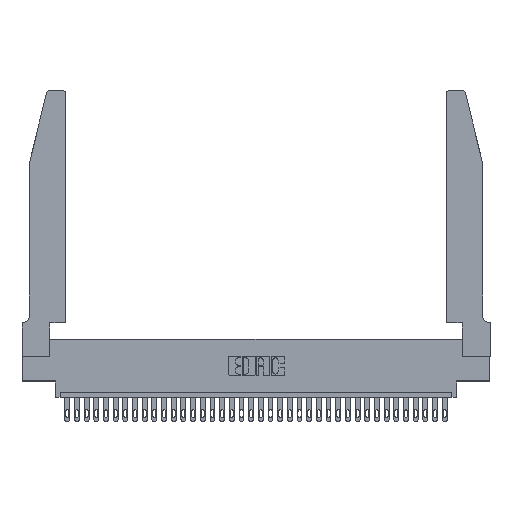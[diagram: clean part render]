
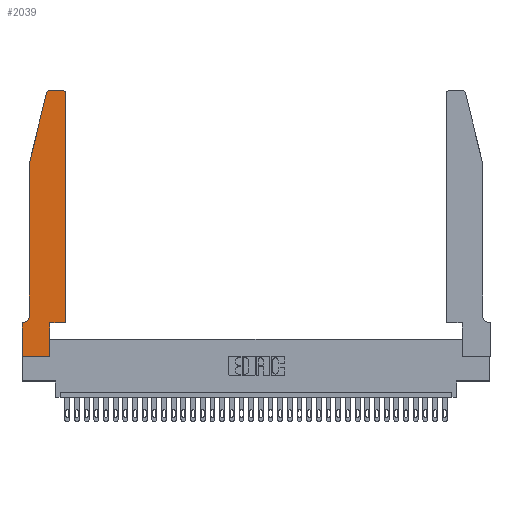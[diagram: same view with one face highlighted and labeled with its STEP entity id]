
A CAD part, top view. The second image highlights one B-rep face of the part: STEP entity #2039.
In plain terms, the highlighted planar face has unit normal (0, 0, 1).
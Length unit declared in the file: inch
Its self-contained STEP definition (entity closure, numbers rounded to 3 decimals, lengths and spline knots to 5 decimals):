
#316 = LINE ( 'NONE', #12608, #26668 ) ;
#741 = DIRECTION ( 'NONE',  ( 1., 0., 0. ) ) ;
#798 = DIRECTION ( 'NONE',  ( 0., 0., 1. ) ) ;
#1268 = VERTEX_POINT ( 'NONE', #8840 ) ;
#2039 = ADVANCED_FACE ( 'NONE', ( #13222 ), #33910, .T. ) ;
#2262 = EDGE_CURVE ( 'NONE', #23707, #23118, #3059, .T. ) ;
#2344 = CARTESIAN_POINT ( 'NONE',  ( 0.4505, 2.72, 0.37 ) ) ;
#2407 = CIRCLE ( 'NONE', #11731, 0.03 ) ;
#2516 = LINE ( 'NONE', #16921, #28808 ) ;
#2754 = EDGE_CURVE ( 'NONE', #29681, #28949, #15750, .T. ) ;
#2791 = ORIENTED_EDGE ( 'NONE', *, *, #12089, .T. ) ;
#2829 = CARTESIAN_POINT ( 'NONE',  ( 0., 0., 0.37 ) ) ;
#3059 = LINE ( 'NONE', #30527, #8102 ) ;
#4511 = LINE ( 'NONE', #7161, #32981 ) ;
#4590 = DIRECTION ( 'NONE',  ( 0., 0., 1. ) ) ;
#4841 = EDGE_CURVE ( 'NONE', #22587, #20092, #33483, .T. ) ;
#7075 = DIRECTION ( 'NONE',  ( 1., 0., 0. ) ) ;
#7161 = CARTESIAN_POINT ( 'NONE',  ( 0., 0., 0.37 ) ) ;
#8011 = DIRECTION ( 'NONE',  ( -1., 0., 0. ) ) ;
#8050 = VERTEX_POINT ( 'NONE', #22201 ) ;
#8102 = VECTOR ( 'NONE', #741, 39.37008 ) ;
#8840 = CARTESIAN_POINT ( 'NONE',  ( 0.0055, 0.35, 0.37 ) ) ;
#9217 = DIRECTION ( 'NONE',  ( 1., 0., 0. ) ) ;
#10300 = VERTEX_POINT ( 'NONE', #2829 ) ;
#10468 = ORIENTED_EDGE ( 'NONE', *, *, #2262, .T. ) ;
#10842 = EDGE_CURVE ( 'NONE', #23118, #29681, #2516, .T. ) ;
#10985 = ORIENTED_EDGE ( 'NONE', *, *, #14538, .T. ) ;
#11731 = AXIS2_PLACEMENT_3D ( 'NONE', #12635, #4590, #7075 ) ;
#12049 = CARTESIAN_POINT ( 'NONE',  ( 0., 0.35, 0.37 ) ) ;
#12089 = EDGE_CURVE ( 'NONE', #10300, #8050, #4511, .T. ) ;
#12608 = CARTESIAN_POINT ( 'NONE',  ( 0.2865, 0.35, 0.37 ) ) ;
#12635 = CARTESIAN_POINT ( 'NONE',  ( 0.284, 2.72, 0.37 ) ) ;
#12711 = VECTOR ( 'NONE', #31027, 39.37008 ) ;
#12812 = VERTEX_POINT ( 'NONE', #15108 ) ;
#13222 = FACE_OUTER_BOUND ( 'NONE', #23418, .T. ) ;
#14308 = CARTESIAN_POINT ( 'NONE',  ( 0.0755, 2., 0.37 ) ) ;
#14431 = LINE ( 'NONE', #31147, #12711 ) ;
#14538 = EDGE_CURVE ( 'NONE', #28949, #34272, #14431, .T. ) ;
#14582 = CARTESIAN_POINT ( 'NONE',  ( 0.4505, 0.35, 0.37 ) ) ;
#15108 = CARTESIAN_POINT ( 'NONE',  ( 0.25487, 2.72718, 0.37 ) ) ;
#15146 = DIRECTION ( 'NONE',  ( 1., 0., 0. ) ) ;
#15150 = ORIENTED_EDGE ( 'NONE', *, *, #21314, .T. ) ;
#15430 = ORIENTED_EDGE ( 'NONE', *, *, #10842, .T. ) ;
#15750 = CIRCLE ( 'NONE', #27082, 0.03 ) ;
#16168 = VECTOR ( 'NONE', #25564, 39.37008 ) ;
#16921 = CARTESIAN_POINT ( 'NONE',  ( 0.4505, 0.35, 0.37 ) ) ;
#17505 = LINE ( 'NONE', #23309, #23835 ) ;
#17812 = ORIENTED_EDGE ( 'NONE', *, *, #4841, .T. ) ;
#17859 = CIRCLE ( 'NONE', #22030, 0.07 ) ;
#18439 = CARTESIAN_POINT ( 'NONE',  ( 0.4205, 2.75, 0.37 ) ) ;
#19090 = CARTESIAN_POINT ( 'NONE',  ( 0.4205, 2.72, 0.37 ) ) ;
#19820 = ORIENTED_EDGE ( 'NONE', *, *, #34894, .T. ) ;
#20049 = CARTESIAN_POINT ( 'NONE',  ( 0., 0.35, 0.37 ) ) ;
#20092 = VERTEX_POINT ( 'NONE', #31010 ) ;
#20788 = EDGE_CURVE ( 'NONE', #30484, #10300, #25074, .T. ) ;
#21314 = EDGE_CURVE ( 'NONE', #20092, #1268, #17859, .T. ) ;
#22030 = AXIS2_PLACEMENT_3D ( 'NONE', #27534, #33015, #30624 ) ;
#22201 = CARTESIAN_POINT ( 'NONE',  ( 0.2865, 0., 0.37 ) ) ;
#22587 = VERTEX_POINT ( 'NONE', #14308 ) ;
#22857 = EDGE_CURVE ( 'NONE', #8050, #23707, #316, .T. ) ;
#23118 = VERTEX_POINT ( 'NONE', #14582 ) ;
#23309 = CARTESIAN_POINT ( 'NONE',  ( 0.0755, 2., 0.37 ) ) ;
#23418 = EDGE_LOOP ( 'NONE', ( #10985, #19820, #28582, #17812, #15150, #25640, #26458, #2791, #25062, #10468, #15430, #31553 ) ) ;
#23707 = VERTEX_POINT ( 'NONE', #33462 ) ;
#23835 = VECTOR ( 'NONE', #28988, 39.37008 ) ;
#24088 = EDGE_CURVE ( 'NONE', #1268, #30484, #24875, .T. ) ;
#24875 = LINE ( 'NONE', #29742, #27831 ) ;
#25062 = ORIENTED_EDGE ( 'NONE', *, *, #22857, .T. ) ;
#25074 = LINE ( 'NONE', #33638, #16168 ) ;
#25078 = DIRECTION ( 'NONE',  ( 0., 1., 0. ) ) ;
#25496 = AXIS2_PLACEMENT_3D ( 'NONE', #12049, #798, #9217 ) ;
#25564 = DIRECTION ( 'NONE',  ( 0., -1., 0. ) ) ;
#25640 = ORIENTED_EDGE ( 'NONE', *, *, #24088, .T. ) ;
#26458 = ORIENTED_EDGE ( 'NONE', *, *, #20788, .T. ) ;
#26504 = CARTESIAN_POINT ( 'NONE',  ( 0.0755, 2., 0.37 ) ) ;
#26668 = VECTOR ( 'NONE', #28989, 39.37008 ) ;
#26827 = DIRECTION ( 'NONE',  ( 0., 0., 1. ) ) ;
#27082 = AXIS2_PLACEMENT_3D ( 'NONE', #19090, #26827, #27160 ) ;
#27093 = VECTOR ( 'NONE', #28981, 39.37008 ) ;
#27160 = DIRECTION ( 'NONE',  ( 1., 0., 0. ) ) ;
#27534 = CARTESIAN_POINT ( 'NONE',  ( 0.0055, 0.42, 0.37 ) ) ;
#27831 = VECTOR ( 'NONE', #8011, 39.37008 ) ;
#28582 = ORIENTED_EDGE ( 'NONE', *, *, #32061, .T. ) ;
#28808 = VECTOR ( 'NONE', #25078, 39.37008 ) ;
#28949 = VERTEX_POINT ( 'NONE', #18439 ) ;
#28981 = DIRECTION ( 'NONE',  ( 0., -1., 0. ) ) ;
#28988 = DIRECTION ( 'NONE',  ( -0.239, -0.971, 0. ) ) ;
#28989 = DIRECTION ( 'NONE',  ( 0., 1., 0. ) ) ;
#29681 = VERTEX_POINT ( 'NONE', #2344 ) ;
#29742 = CARTESIAN_POINT ( 'NONE',  ( 0.0755, 0.35, 0.37 ) ) ;
#30484 = VERTEX_POINT ( 'NONE', #20049 ) ;
#30527 = CARTESIAN_POINT ( 'NONE',  ( 0.4505, 0.35, 0.37 ) ) ;
#30624 = DIRECTION ( 'NONE',  ( -1., 0., 0. ) ) ;
#31010 = CARTESIAN_POINT ( 'NONE',  ( 0.0755, 0.42, 0.37 ) ) ;
#31027 = DIRECTION ( 'NONE',  ( -1., 0., 0. ) ) ;
#31147 = CARTESIAN_POINT ( 'NONE',  ( 0.2605, 2.75, 0.37 ) ) ;
#31553 = ORIENTED_EDGE ( 'NONE', *, *, #2754, .T. ) ;
#32061 = EDGE_CURVE ( 'NONE', #12812, #22587, #17505, .T. ) ;
#32981 = VECTOR ( 'NONE', #15146, 39.37008 ) ;
#33015 = DIRECTION ( 'NONE',  ( 0., 0., -1. ) ) ;
#33259 = CARTESIAN_POINT ( 'NONE',  ( 0.284, 2.75, 0.37 ) ) ;
#33462 = CARTESIAN_POINT ( 'NONE',  ( 0.2865, 0.35, 0.37 ) ) ;
#33483 = LINE ( 'NONE', #26504, #27093 ) ;
#33638 = CARTESIAN_POINT ( 'NONE',  ( 0., 0., 0.37 ) ) ;
#33910 = PLANE ( 'NONE',  #25496 ) ;
#34272 = VERTEX_POINT ( 'NONE', #33259 ) ;
#34894 = EDGE_CURVE ( 'NONE', #34272, #12812, #2407, .T. ) ;
